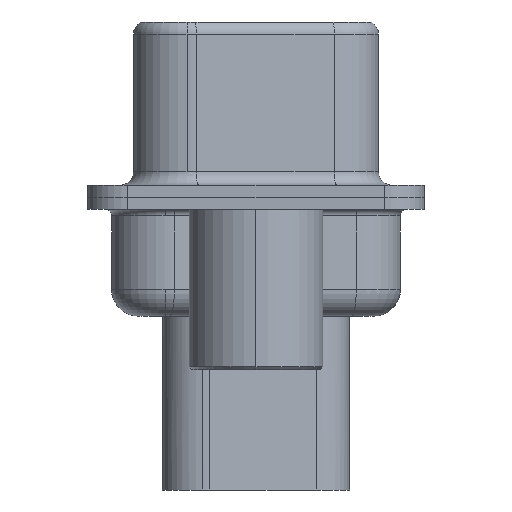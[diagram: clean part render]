
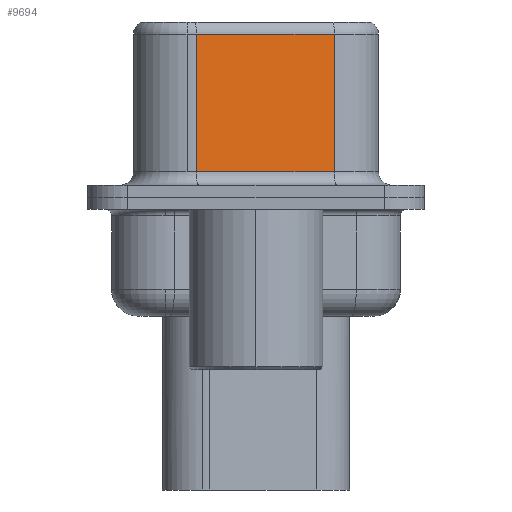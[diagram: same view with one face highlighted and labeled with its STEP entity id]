
A CAD part, left-side view. The second image highlights one B-rep face of the part: STEP entity #9694.
In plain terms, the highlighted planar face has unit normal (-0.985, -0.174, 0).
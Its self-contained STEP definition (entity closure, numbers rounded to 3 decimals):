
#450 = DIRECTION ( 'NONE',  ( -0.174, 0.985, 0. ) ) ;
#970 = EDGE_CURVE ( 'NONE', #2679, #9784, #5402, .T. ) ;
#1040 = VERTEX_POINT ( 'NONE', #10250 ) ;
#1626 = CARTESIAN_POINT ( 'NONE',  ( 4.575, -2.927, 0.95 ) ) ;
#1631 = EDGE_CURVE ( 'NONE', #1040, #2679, #3674, .T. ) ;
#1904 = CARTESIAN_POINT ( 'NONE',  ( 4.575, -2.927, 6.55 ) ) ;
#1973 = DIRECTION ( 'NONE',  ( 0., 0., -1. ) ) ;
#2021 = AXIS2_PLACEMENT_3D ( 'NONE', #11326, #11256, #450 ) ;
#2022 = VECTOR ( 'NONE', #1973, 1000. ) ;
#2349 = FACE_OUTER_BOUND ( 'NONE', #3586, .T. ) ;
#2679 = VERTEX_POINT ( 'NONE', #12061 ) ;
#2701 = CARTESIAN_POINT ( 'NONE',  ( 4.575, -2.927, 6.1 ) ) ;
#2716 = VERTEX_POINT ( 'NONE', #12188 ) ;
#3026 = VECTOR ( 'NONE', #3755, 1000. ) ;
#3586 = EDGE_LOOP ( 'NONE', ( #10515, #4159, #11777, #8937 ) ) ;
#3674 = LINE ( 'NONE', #2701, #8760 ) ;
#3755 = DIRECTION ( 'NONE',  ( 0.174, -0.985, 0. ) ) ;
#4159 = ORIENTED_EDGE ( 'NONE', *, *, #1631, .T. ) ;
#5402 = LINE ( 'NONE', #6246, #6967 ) ;
#5620 = CARTESIAN_POINT ( 'NONE',  ( 3.665, 2.233, 0.95 ) ) ;
#6246 = CARTESIAN_POINT ( 'NONE',  ( 3.665, 2.233, 6.55 ) ) ;
#6967 = VECTOR ( 'NONE', #9290, 1000. ) ;
#7886 = EDGE_CURVE ( 'NONE', #9784, #2716, #10544, .T. ) ;
#7924 = LINE ( 'NONE', #1904, #2022 ) ;
#8299 = PLANE ( 'NONE',  #2021 ) ;
#8760 = VECTOR ( 'NONE', #11741, 1000. ) ;
#8937 = ORIENTED_EDGE ( 'NONE', *, *, #7886, .T. ) ;
#9290 = DIRECTION ( 'NONE',  ( 0., 0., -1. ) ) ;
#9694 = ADVANCED_FACE ( 'NONE', ( #2349 ), #8299, .F. ) ;
#9784 = VERTEX_POINT ( 'NONE', #5620 ) ;
#10250 = CARTESIAN_POINT ( 'NONE',  ( 4.575, -2.927, 6.1 ) ) ;
#10515 = ORIENTED_EDGE ( 'NONE', *, *, #12679, .F. ) ;
#10544 = LINE ( 'NONE', #1626, #3026 ) ;
#11256 = DIRECTION ( 'NONE',  ( 0.985, 0.174, 0. ) ) ;
#11326 = CARTESIAN_POINT ( 'NONE',  ( 4.575, -2.927, 6.55 ) ) ;
#11741 = DIRECTION ( 'NONE',  ( -0.174, 0.985, 0. ) ) ;
#11777 = ORIENTED_EDGE ( 'NONE', *, *, #970, .T. ) ;
#12061 = CARTESIAN_POINT ( 'NONE',  ( 3.665, 2.233, 6.1 ) ) ;
#12188 = CARTESIAN_POINT ( 'NONE',  ( 4.575, -2.927, 0.95 ) ) ;
#12679 = EDGE_CURVE ( 'NONE', #1040, #2716, #7924, .T. ) ;
